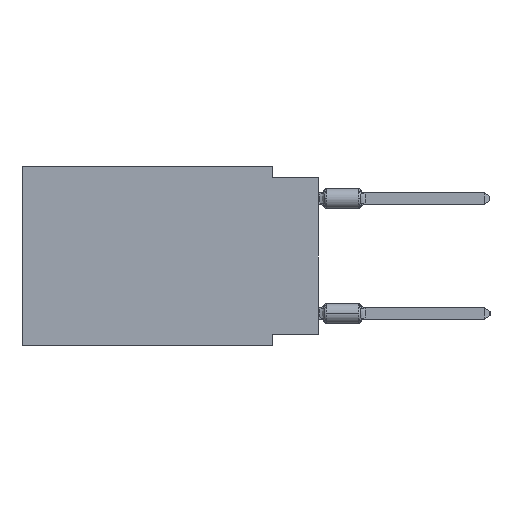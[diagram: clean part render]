
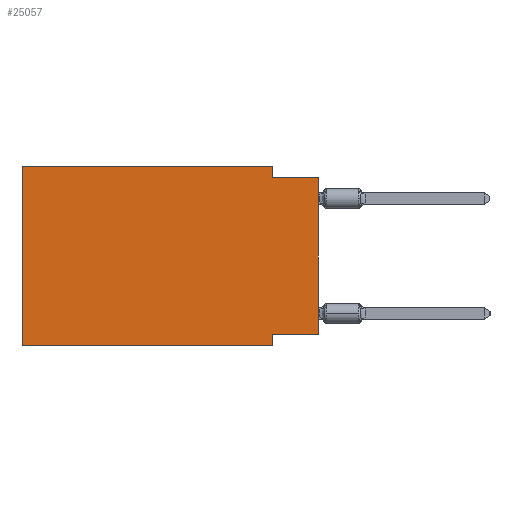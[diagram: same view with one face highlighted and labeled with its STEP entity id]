
A CAD part, left-side view. The second image highlights one B-rep face of the part: STEP entity #25057.
In plain terms, the highlighted planar face has unit normal (-1, 0, 0).
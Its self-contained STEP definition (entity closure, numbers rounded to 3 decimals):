
#236 = CARTESIAN_POINT ( 'NONE',  ( 0., 0., -0.635 ) ) ;
#550 = VERTEX_POINT ( 'NONE', #56856 ) ;
#986 = VERTEX_POINT ( 'NONE', #4594 ) ;
#1117 = ORIENTED_EDGE ( 'NONE', *, *, #28433, .F. ) ;
#3520 = VECTOR ( 'NONE', #29318, 1000. ) ;
#4594 = CARTESIAN_POINT ( 'NONE',  ( 0., 0., -0.635 ) ) ;
#5408 = DIRECTION ( 'NONE',  ( 0., -1., 0. ) ) ;
#5704 = ORIENTED_EDGE ( 'NONE', *, *, #38043, .F. ) ;
#7323 = DIRECTION ( 'NONE',  ( 0., 0., -1. ) ) ;
#8790 = VERTEX_POINT ( 'NONE', #32449 ) ;
#10721 = LINE ( 'NONE', #54011, #56376 ) ;
#11826 = LINE ( 'NONE', #13077, #38373 ) ;
#13077 = CARTESIAN_POINT ( 'NONE',  ( 0., 16.383, 0. ) ) ;
#13723 = LINE ( 'NONE', #236, #35927 ) ;
#14187 = CARTESIAN_POINT ( 'NONE',  ( 0., 16.383, 0. ) ) ;
#15361 = VECTOR ( 'NONE', #56332, 1000. ) ;
#17168 = EDGE_CURVE ( 'NONE', #48246, #550, #40883, .T. ) ;
#17380 = EDGE_CURVE ( 'NONE', #58598, #21249, #10721, .T. ) ;
#18289 = EDGE_CURVE ( 'NONE', #21249, #8790, #21438, .T. ) ;
#19199 = DIRECTION ( 'NONE',  ( 0., 0., -1. ) ) ;
#21055 = CARTESIAN_POINT ( 'NONE',  ( 0., 2.54, 0. ) ) ;
#21249 = VERTEX_POINT ( 'NONE', #21055 ) ;
#21438 = LINE ( 'NONE', #41525, #52414 ) ;
#22724 = LINE ( 'NONE', #37172, #15361 ) ;
#22744 = DIRECTION ( 'NONE',  ( 0., -1., 0. ) ) ;
#25057 = ADVANCED_FACE ( 'NONE', ( #38035 ), #57200, .F. ) ;
#25165 = CARTESIAN_POINT ( 'NONE',  ( 0., 2.54, -9.906 ) ) ;
#25876 = AXIS2_PLACEMENT_3D ( 'NONE', #14187, #33326, #19199 ) ;
#26120 = CARTESIAN_POINT ( 'NONE',  ( 0., 0., -9.271 ) ) ;
#26767 = EDGE_CURVE ( 'NONE', #8790, #986, #13723, .T. ) ;
#28433 = EDGE_CURVE ( 'NONE', #550, #37472, #47222, .T. ) ;
#29318 = DIRECTION ( 'NONE',  ( 0., 0., -1. ) ) ;
#29388 = DIRECTION ( 'NONE',  ( 0., -1., 0. ) ) ;
#30341 = ORIENTED_EDGE ( 'NONE', *, *, #44605, .T. ) ;
#30846 = CARTESIAN_POINT ( 'NONE',  ( 0., 0., -9.271 ) ) ;
#31476 = DIRECTION ( 'NONE',  ( 0., 1., 0. ) ) ;
#32225 = DIRECTION ( 'NONE',  ( 0., 0., 1. ) ) ;
#32265 = VECTOR ( 'NONE', #31476, 1000. ) ;
#32449 = CARTESIAN_POINT ( 'NONE',  ( 0., 2.54, -0.635 ) ) ;
#33326 = DIRECTION ( 'NONE',  ( 1., 0., 0. ) ) ;
#35424 = ORIENTED_EDGE ( 'NONE', *, *, #17380, .F. ) ;
#35927 = VECTOR ( 'NONE', #29388, 1000. ) ;
#37172 = CARTESIAN_POINT ( 'NONE',  ( 0., 0., 0. ) ) ;
#37472 = VERTEX_POINT ( 'NONE', #25165 ) ;
#38035 = FACE_OUTER_BOUND ( 'NONE', #61958, .T. ) ;
#38043 = EDGE_CURVE ( 'NONE', #61718, #58598, #11826, .T. ) ;
#38373 = VECTOR ( 'NONE', #32225, 1000. ) ;
#38600 = ORIENTED_EDGE ( 'NONE', *, *, #48044, .T. ) ;
#40883 = LINE ( 'NONE', #30846, #32265 ) ;
#41525 = CARTESIAN_POINT ( 'NONE',  ( 0., 2.54, 0. ) ) ;
#42823 = LINE ( 'NONE', #47527, #52731 ) ;
#44605 = EDGE_CURVE ( 'NONE', #48246, #986, #22724, .T. ) ;
#45364 = CARTESIAN_POINT ( 'NONE',  ( 0., 16.383, 0. ) ) ;
#45732 = ORIENTED_EDGE ( 'NONE', *, *, #17168, .F. ) ;
#47175 = ORIENTED_EDGE ( 'NONE', *, *, #26767, .F. ) ;
#47222 = LINE ( 'NONE', #57598, #3520 ) ;
#47527 = CARTESIAN_POINT ( 'NONE',  ( 0., 16.383, -9.906 ) ) ;
#47789 = CARTESIAN_POINT ( 'NONE',  ( 0., 16.383, -9.906 ) ) ;
#48044 = EDGE_CURVE ( 'NONE', #61718, #37472, #42823, .T. ) ;
#48246 = VERTEX_POINT ( 'NONE', #26120 ) ;
#52414 = VECTOR ( 'NONE', #7323, 1000. ) ;
#52731 = VECTOR ( 'NONE', #22744, 1000. ) ;
#53405 = ORIENTED_EDGE ( 'NONE', *, *, #18289, .F. ) ;
#54011 = CARTESIAN_POINT ( 'NONE',  ( 0., 16.383, 0. ) ) ;
#56332 = DIRECTION ( 'NONE',  ( 0., 0., 1. ) ) ;
#56376 = VECTOR ( 'NONE', #5408, 1000. ) ;
#56856 = CARTESIAN_POINT ( 'NONE',  ( 0., 2.54, -9.271 ) ) ;
#57200 = PLANE ( 'NONE',  #25876 ) ;
#57598 = CARTESIAN_POINT ( 'NONE',  ( 0., 2.54, -9.906 ) ) ;
#58598 = VERTEX_POINT ( 'NONE', #45364 ) ;
#61718 = VERTEX_POINT ( 'NONE', #47789 ) ;
#61958 = EDGE_LOOP ( 'NONE', ( #30341, #47175, #53405, #35424, #5704, #38600, #1117, #45732 ) ) ;
